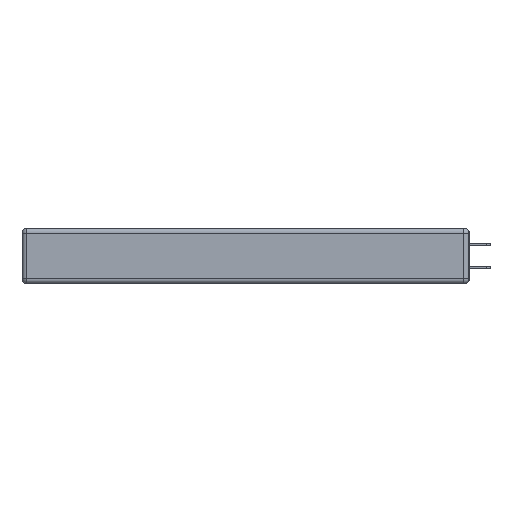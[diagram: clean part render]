
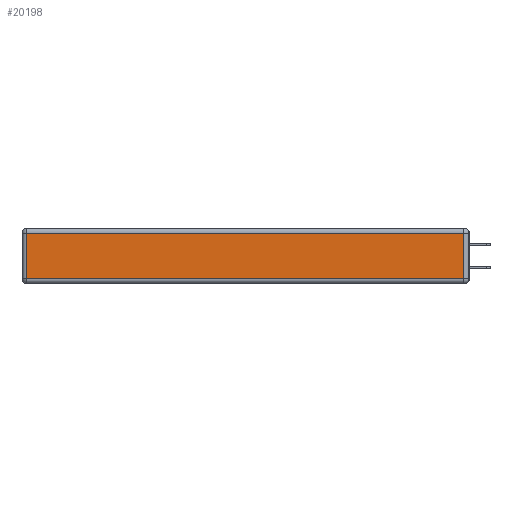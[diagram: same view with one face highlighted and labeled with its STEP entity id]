
A CAD part, left-side view. The second image highlights one B-rep face of the part: STEP entity #20198.
In plain terms, the highlighted planar face has unit normal (-1, 0, 0).
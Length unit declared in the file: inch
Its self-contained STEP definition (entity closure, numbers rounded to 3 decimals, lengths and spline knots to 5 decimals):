
#375 = CARTESIAN_POINT ( 'NONE',  ( 0., 2.72, -0.03 ) ) ;
#884 = DIRECTION ( 'NONE',  ( 0., 0., -1. ) ) ;
#1089 = CARTESIAN_POINT ( 'NONE',  ( 0., 0., -0.343 ) ) ;
#1659 = ORIENTED_EDGE ( 'NONE', *, *, #8142, .T. ) ;
#2262 = VERTEX_POINT ( 'NONE', #7166 ) ;
#2561 = DIRECTION ( 'NONE',  ( 0., -1., 0. ) ) ;
#3143 = CARTESIAN_POINT ( 'NONE',  ( 0., 2.72, -0.343 ) ) ;
#3615 = ORIENTED_EDGE ( 'NONE', *, *, #11908, .T. ) ;
#4446 = EDGE_CURVE ( 'NONE', #15235, #2262, #9915, .T. ) ;
#7166 = CARTESIAN_POINT ( 'NONE',  ( 0., 0.03, -0.313 ) ) ;
#7902 = AXIS2_PLACEMENT_3D ( 'NONE', #1089, #20887, #18158 ) ;
#8142 = EDGE_CURVE ( 'NONE', #13512, #15921, #18306, .T. ) ;
#8222 = CARTESIAN_POINT ( 'NONE',  ( 0., 0.03, -0.343 ) ) ;
#9915 = LINE ( 'NONE', #12645, #27913 ) ;
#11803 = ORIENTED_EDGE ( 'NONE', *, *, #19412, .T. ) ;
#11812 = VECTOR ( 'NONE', #20060, 39.37008 ) ;
#11908 = EDGE_CURVE ( 'NONE', #2262, #13512, #12589, .T. ) ;
#12589 = LINE ( 'NONE', #8222, #29119 ) ;
#12645 = CARTESIAN_POINT ( 'NONE',  ( 0., 0., -0.313 ) ) ;
#13512 = VERTEX_POINT ( 'NONE', #16081 ) ;
#15235 = VERTEX_POINT ( 'NONE', #19150 ) ;
#15921 = VERTEX_POINT ( 'NONE', #375 ) ;
#16081 = CARTESIAN_POINT ( 'NONE',  ( 0., 0.03, -0.03 ) ) ;
#16611 = LINE ( 'NONE', #3143, #28163 ) ;
#17993 = DIRECTION ( 'NONE',  ( 0., 0., 1. ) ) ;
#18158 = DIRECTION ( 'NONE',  ( 0., 0., 1. ) ) ;
#18306 = LINE ( 'NONE', #18874, #11812 ) ;
#18847 = FACE_OUTER_BOUND ( 'NONE', #25854, .T. ) ;
#18874 = CARTESIAN_POINT ( 'NONE',  ( 0., 2.75, -0.03 ) ) ;
#19150 = CARTESIAN_POINT ( 'NONE',  ( 0., 2.72, -0.313 ) ) ;
#19412 = EDGE_CURVE ( 'NONE', #15921, #15235, #16611, .T. ) ;
#20060 = DIRECTION ( 'NONE',  ( 0., 1., 0. ) ) ;
#20198 = ADVANCED_FACE ( 'NONE', ( #18847 ), #25590, .T. ) ;
#20562 = ORIENTED_EDGE ( 'NONE', *, *, #4446, .T. ) ;
#20887 = DIRECTION ( 'NONE',  ( -1., 0., 0. ) ) ;
#25590 = PLANE ( 'NONE',  #7902 ) ;
#25854 = EDGE_LOOP ( 'NONE', ( #20562, #3615, #1659, #11803 ) ) ;
#27913 = VECTOR ( 'NONE', #2561, 39.37008 ) ;
#28163 = VECTOR ( 'NONE', #884, 39.37008 ) ;
#29119 = VECTOR ( 'NONE', #17993, 39.37008 ) ;
